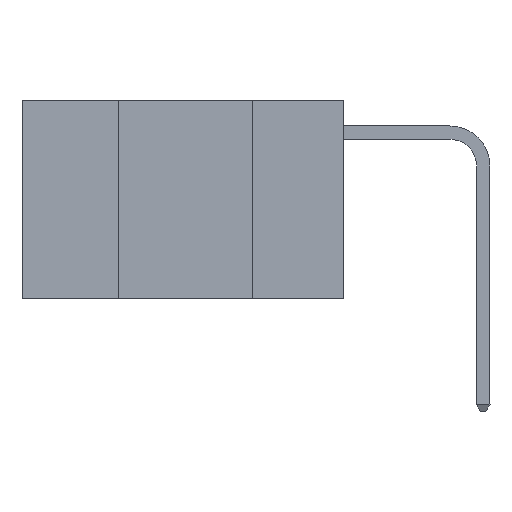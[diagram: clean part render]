
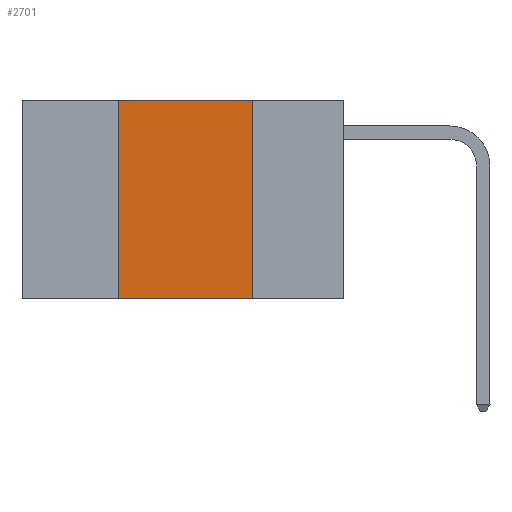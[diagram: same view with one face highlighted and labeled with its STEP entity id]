
A CAD part, left-side view. The second image highlights one B-rep face of the part: STEP entity #2701.
In plain terms, the highlighted planar face has unit normal (-1, 0, 0).
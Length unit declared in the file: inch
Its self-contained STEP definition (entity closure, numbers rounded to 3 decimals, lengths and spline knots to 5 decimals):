
#54 = VECTOR ( 'NONE', #10434, 39.37008 ) ;
#465 = EDGE_CURVE ( 'NONE', #16841, #15668, #6674, .T. ) ;
#673 = ORIENTED_EDGE ( 'NONE', *, *, #2783, .F. ) ;
#1304 = DIRECTION ( 'NONE',  ( 0., -1., 0. ) ) ;
#1699 = EDGE_CURVE ( 'NONE', #16841, #15796, #18534, .T. ) ;
#1920 = ORIENTED_EDGE ( 'NONE', *, *, #465, .T. ) ;
#2219 = CARTESIAN_POINT ( 'NONE',  ( 0., 0.17, -0.37 ) ) ;
#2701 = ADVANCED_FACE ( 'NONE', ( #19895 ), #19210, .F. ) ;
#2783 = EDGE_CURVE ( 'NONE', #15796, #5123, #22903, .T. ) ;
#3150 = CARTESIAN_POINT ( 'NONE',  ( 0., 0.6, 0. ) ) ;
#3517 = VECTOR ( 'NONE', #11481, 39.37008 ) ;
#3749 = VECTOR ( 'NONE', #1304, 39.37008 ) ;
#4741 = ORIENTED_EDGE ( 'NONE', *, *, #5348, .F. ) ;
#5123 = VERTEX_POINT ( 'NONE', #18791 ) ;
#5348 = EDGE_CURVE ( 'NONE', #5123, #15668, #15168, .T. ) ;
#5810 = CARTESIAN_POINT ( 'NONE',  ( 0., 0.42, -0.37 ) ) ;
#6674 = LINE ( 'NONE', #11796, #15821 ) ;
#7022 = ORIENTED_EDGE ( 'NONE', *, *, #1699, .F. ) ;
#8377 = CARTESIAN_POINT ( 'NONE',  ( 0., 0.6, 0. ) ) ;
#10064 = EDGE_LOOP ( 'NONE', ( #4741, #673, #7022, #1920 ) ) ;
#10220 = DIRECTION ( 'NONE',  ( 1., 0., 0. ) ) ;
#10434 = DIRECTION ( 'NONE',  ( 0., 0., -1. ) ) ;
#11481 = DIRECTION ( 'NONE',  ( 0., 0., 1. ) ) ;
#11796 = CARTESIAN_POINT ( 'NONE',  ( 0., 0.6, -0.37 ) ) ;
#11829 = CARTESIAN_POINT ( 'NONE',  ( 0., 0.42, 0. ) ) ;
#11881 = DIRECTION ( 'NONE',  ( 0., -1., 0. ) ) ;
#13522 = AXIS2_PLACEMENT_3D ( 'NONE', #8377, #10220, #22759 ) ;
#14104 = CARTESIAN_POINT ( 'NONE',  ( 0., 0.17, 0. ) ) ;
#15168 = LINE ( 'NONE', #14104, #54 ) ;
#15668 = VERTEX_POINT ( 'NONE', #2219 ) ;
#15796 = VERTEX_POINT ( 'NONE', #20627 ) ;
#15821 = VECTOR ( 'NONE', #11881, 39.37008 ) ;
#16841 = VERTEX_POINT ( 'NONE', #5810 ) ;
#18534 = LINE ( 'NONE', #11829, #3517 ) ;
#18791 = CARTESIAN_POINT ( 'NONE',  ( 0., 0.17, 0. ) ) ;
#19210 = PLANE ( 'NONE',  #13522 ) ;
#19895 = FACE_OUTER_BOUND ( 'NONE', #10064, .T. ) ;
#20627 = CARTESIAN_POINT ( 'NONE',  ( 0., 0.42, 0. ) ) ;
#22759 = DIRECTION ( 'NONE',  ( 0., 0., -1. ) ) ;
#22903 = LINE ( 'NONE', #3150, #3749 ) ;
